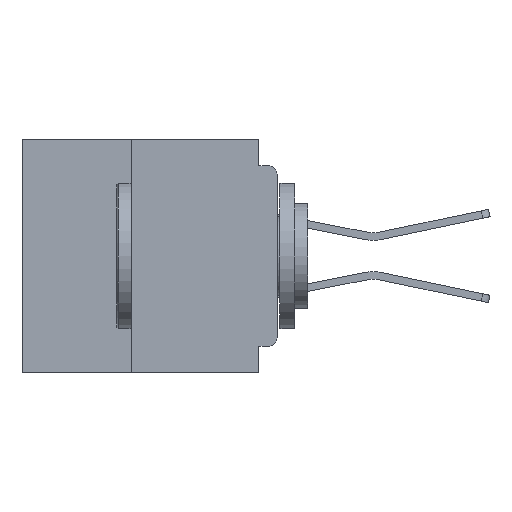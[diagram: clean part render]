
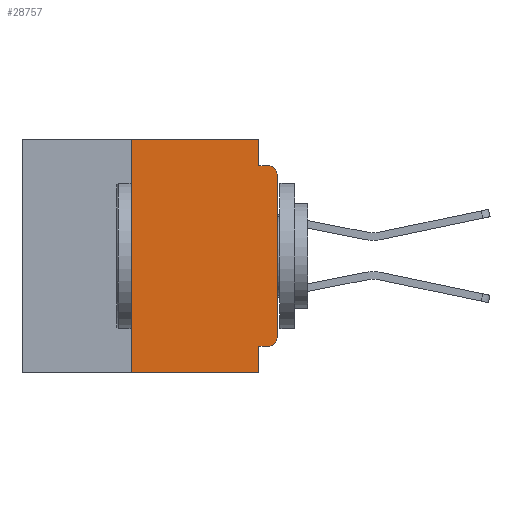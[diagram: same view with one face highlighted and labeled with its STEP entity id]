
A CAD part, left-side view. The second image highlights one B-rep face of the part: STEP entity #28757.
In plain terms, the highlighted planar face has unit normal (-1, 0, 0).
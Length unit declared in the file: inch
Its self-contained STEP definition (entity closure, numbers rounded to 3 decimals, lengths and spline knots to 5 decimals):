
#855 = VECTOR ( 'NONE', #7606, 39.37008 ) ;
#2043 = CARTESIAN_POINT ( 'NONE',  ( 0., 0.015, -0.34 ) ) ;
#2492 = AXIS2_PLACEMENT_3D ( 'NONE', #16946, #41332, #20568 ) ;
#3326 = EDGE_CURVE ( 'NONE', #14273, #5791, #6902, .T. ) ;
#3394 = DIRECTION ( 'NONE',  ( 0., 0., -1. ) ) ;
#4703 = EDGE_CURVE ( 'NONE', #5791, #37527, #39802, .T. ) ;
#4792 = CARTESIAN_POINT ( 'NONE',  ( 0., 0.25, -0.4 ) ) ;
#5667 = DIRECTION ( 'NONE',  ( 0., 0., -1. ) ) ;
#5749 = VECTOR ( 'NONE', #7734, 39.37008 ) ;
#5791 = VERTEX_POINT ( 'NONE', #37000 ) ;
#5829 = LINE ( 'NONE', #18217, #42129 ) ;
#6415 = VERTEX_POINT ( 'NONE', #11818 ) ;
#6699 = VERTEX_POINT ( 'NONE', #37715 ) ;
#6902 = LINE ( 'NONE', #10463, #5749 ) ;
#7606 = DIRECTION ( 'NONE',  ( 0., 0., 1. ) ) ;
#7734 = DIRECTION ( 'NONE',  ( 0., 1., 0. ) ) ;
#7998 = LINE ( 'NONE', #26686, #25846 ) ;
#8017 = EDGE_CURVE ( 'NONE', #6699, #8307, #34703, .T. ) ;
#8307 = VERTEX_POINT ( 'NONE', #29154 ) ;
#8974 = CARTESIAN_POINT ( 'NONE',  ( 0., 0.25, 0. ) ) ;
#9483 = ORIENTED_EDGE ( 'NONE', *, *, #29885, .F. ) ;
#10463 = CARTESIAN_POINT ( 'NONE',  ( 0., 0., -0.355 ) ) ;
#10714 = VECTOR ( 'NONE', #30621, 39.37008 ) ;
#11286 = EDGE_CURVE ( 'NONE', #17718, #37527, #24282, .T. ) ;
#11517 = VERTEX_POINT ( 'NONE', #35723 ) ;
#11673 = LINE ( 'NONE', #43258, #21178 ) ;
#11818 = CARTESIAN_POINT ( 'NONE',  ( 0., 0.031, 0. ) ) ;
#12060 = AXIS2_PLACEMENT_3D ( 'NONE', #41992, #24794, #3394 ) ;
#12368 = EDGE_CURVE ( 'NONE', #6415, #24013, #7998, .T. ) ;
#13061 = ORIENTED_EDGE ( 'NONE', *, *, #11286, .T. ) ;
#14273 = VERTEX_POINT ( 'NONE', #23331 ) ;
#14964 = FACE_OUTER_BOUND ( 'NONE', #33315, .T. ) ;
#14990 = CARTESIAN_POINT ( 'NONE',  ( 0., 0.25, -0.4 ) ) ;
#16848 = CARTESIAN_POINT ( 'NONE',  ( 0., 0.031, -0.045 ) ) ;
#16946 = CARTESIAN_POINT ( 'NONE',  ( 0., 0.015, -0.06 ) ) ;
#17718 = VERTEX_POINT ( 'NONE', #4792 ) ;
#18217 = CARTESIAN_POINT ( 'NONE',  ( 0., 0.437, 0. ) ) ;
#20568 = DIRECTION ( 'NONE',  ( 0., 0., -1. ) ) ;
#21178 = VECTOR ( 'NONE', #36388, 39.37008 ) ;
#21202 = EDGE_CURVE ( 'NONE', #24013, #8307, #35955, .T. ) ;
#21715 = ORIENTED_EDGE ( 'NONE', *, *, #3326, .F. ) ;
#22470 = ORIENTED_EDGE ( 'NONE', *, *, #21202, .F. ) ;
#22886 = EDGE_CURVE ( 'NONE', #14273, #11517, #38623, .T. ) ;
#23331 = CARTESIAN_POINT ( 'NONE',  ( 0., 0.015, -0.355 ) ) ;
#23352 = EDGE_CURVE ( 'NONE', #11517, #6699, #11673, .T. ) ;
#23458 = DIRECTION ( 'NONE',  ( 0., -1., 0. ) ) ;
#24013 = VERTEX_POINT ( 'NONE', #16848 ) ;
#24251 = ORIENTED_EDGE ( 'NONE', *, *, #12368, .F. ) ;
#24282 = LINE ( 'NONE', #40683, #41574 ) ;
#24288 = EDGE_CURVE ( 'NONE', #17718, #42228, #40615, .T. ) ;
#24794 = DIRECTION ( 'NONE',  ( 1., 0., 0. ) ) ;
#25375 = DIRECTION ( 'NONE',  ( 0., -1., 0. ) ) ;
#25846 = VECTOR ( 'NONE', #30180, 39.37008 ) ;
#26686 = CARTESIAN_POINT ( 'NONE',  ( 0., 0.031, 0. ) ) ;
#26788 = ORIENTED_EDGE ( 'NONE', *, *, #8017, .T. ) ;
#27039 = DIRECTION ( 'NONE',  ( -1., 0., 0. ) ) ;
#27097 = ORIENTED_EDGE ( 'NONE', *, *, #4703, .F. ) ;
#27333 = AXIS2_PLACEMENT_3D ( 'NONE', #2043, #27039, #5667 ) ;
#27811 = DIRECTION ( 'NONE',  ( 0., -1., 0. ) ) ;
#28158 = PLANE ( 'NONE',  #12060 ) ;
#28693 = CARTESIAN_POINT ( 'NONE',  ( 0., 0.031, -0.4 ) ) ;
#28757 = ADVANCED_FACE ( 'NONE', ( #14964 ), #28158, .F. ) ;
#29154 = CARTESIAN_POINT ( 'NONE',  ( 0., 0.015, -0.045 ) ) ;
#29802 = ORIENTED_EDGE ( 'NONE', *, *, #22886, .T. ) ;
#29885 = EDGE_CURVE ( 'NONE', #42228, #6415, #5829, .T. ) ;
#30180 = DIRECTION ( 'NONE',  ( 0., 0., -1. ) ) ;
#30621 = DIRECTION ( 'NONE',  ( 0., 0., -1. ) ) ;
#33315 = EDGE_LOOP ( 'NONE', ( #38726, #26788, #22470, #24251, #9483, #40778, #13061, #27097, #21715, #29802 ) ) ;
#34595 = CARTESIAN_POINT ( 'NONE',  ( 0., 0., -0.045 ) ) ;
#34703 = CIRCLE ( 'NONE', #2492, 0.015 ) ;
#34862 = VECTOR ( 'NONE', #27811, 39.37008 ) ;
#35723 = CARTESIAN_POINT ( 'NONE',  ( 0., 0., -0.34 ) ) ;
#35955 = LINE ( 'NONE', #34595, #34862 ) ;
#36388 = DIRECTION ( 'NONE',  ( 0., 0., 1. ) ) ;
#37000 = CARTESIAN_POINT ( 'NONE',  ( 0., 0.031, -0.355 ) ) ;
#37527 = VERTEX_POINT ( 'NONE', #40779 ) ;
#37715 = CARTESIAN_POINT ( 'NONE',  ( 0., 0., -0.06 ) ) ;
#38623 = CIRCLE ( 'NONE', #27333, 0.015 ) ;
#38726 = ORIENTED_EDGE ( 'NONE', *, *, #23352, .T. ) ;
#39802 = LINE ( 'NONE', #28693, #10714 ) ;
#40615 = LINE ( 'NONE', #14990, #855 ) ;
#40683 = CARTESIAN_POINT ( 'NONE',  ( 0., 0.437, -0.4 ) ) ;
#40778 = ORIENTED_EDGE ( 'NONE', *, *, #24288, .F. ) ;
#40779 = CARTESIAN_POINT ( 'NONE',  ( 0., 0.031, -0.4 ) ) ;
#41332 = DIRECTION ( 'NONE',  ( -1., 0., 0. ) ) ;
#41574 = VECTOR ( 'NONE', #23458, 39.37008 ) ;
#41992 = CARTESIAN_POINT ( 'NONE',  ( 0., 0.437, 0. ) ) ;
#42129 = VECTOR ( 'NONE', #25375, 39.37008 ) ;
#42228 = VERTEX_POINT ( 'NONE', #8974 ) ;
#43258 = CARTESIAN_POINT ( 'NONE',  ( 0., 0., 0. ) ) ;
